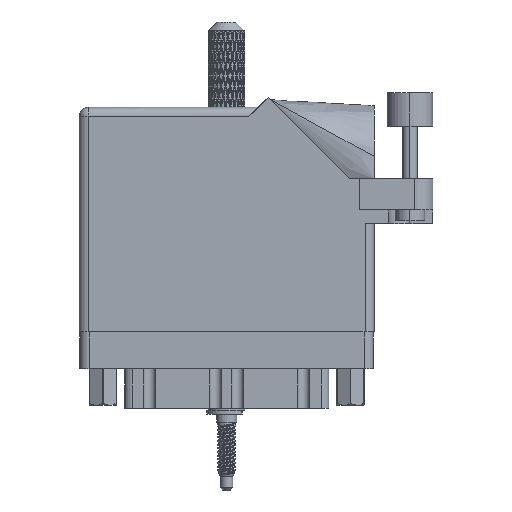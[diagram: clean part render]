
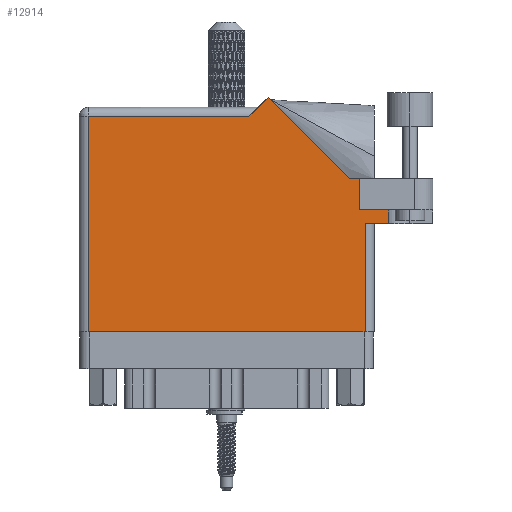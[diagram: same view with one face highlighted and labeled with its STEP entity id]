
A CAD part, front view. The second image highlights one B-rep face of the part: STEP entity #12914.
In plain terms, the highlighted face is planar.
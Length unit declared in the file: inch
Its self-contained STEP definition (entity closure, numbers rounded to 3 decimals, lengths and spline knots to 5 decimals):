
#301 = DIRECTION ( 'NONE',  ( 1., 0., 0. ) ) ;
#381 = ORIENTED_EDGE ( 'NONE', *, *, #11317, .T. ) ;
#4269 = CARTESIAN_POINT ( 'NONE',  ( 0., 1.53, 0. ) ) ;
#4334 = ORIENTED_EDGE ( 'NONE', *, *, #68360, .T. ) ;
#4575 = ORIENTED_EDGE ( 'NONE', *, *, #110889, .T. ) ;
#5026 = DIRECTION ( 'NONE',  ( 0., -1., 0. ) ) ;
#5050 = DIRECTION ( 'NONE',  ( 0., -1., 0. ) ) ;
#5153 = ORIENTED_EDGE ( 'NONE', *, *, #79553, .T. ) ;
#5802 = ORIENTED_EDGE ( 'NONE', *, *, #62195, .T. ) ;
#7744 = DIRECTION ( 'NONE',  ( -1., 0., 0. ) ) ;
#8622 = CARTESIAN_POINT ( 'NONE',  ( 0.062, 0., 0. ) ) ;
#9387 = DIRECTION ( 'NONE',  ( 0., 1., 0. ) ) ;
#10222 = ORIENTED_EDGE ( 'NONE', *, *, #43033, .F. ) ;
#10586 = DIRECTION ( 'NONE',  ( 0., 0., -1. ) ) ;
#11130 = CARTESIAN_POINT ( 'NONE',  ( 2.1115, 0.737, 0. ) ) ;
#11317 = EDGE_CURVE ( 'NONE', #102012, #17183, #24519, .T. ) ;
#11577 = VECTOR ( 'NONE', #9387, 39.37008 ) ;
#11699 = VERTEX_POINT ( 'NONE', #77248 ) ;
#12588 = DIRECTION ( 'NONE',  ( 0., 1., 0. ) ) ;
#12914 = ADVANCED_FACE ( 'NONE', ( #55962 ), #21453, .F. ) ;
#13253 = VECTOR ( 'NONE', #5026, 39.37008 ) ;
#14575 = VERTEX_POINT ( 'NONE', #109642 ) ;
#15927 = CARTESIAN_POINT ( 'NONE',  ( 0.062, 1.468, 0. ) ) ;
#17110 = VERTEX_POINT ( 'NONE', #109288 ) ;
#17183 = VERTEX_POINT ( 'NONE', #22547 ) ;
#17669 = ORIENTED_EDGE ( 'NONE', *, *, #80938, .T. ) ;
#18064 = LINE ( 'NONE', #88179, #62776 ) ;
#20840 = ORIENTED_EDGE ( 'NONE', *, *, #104533, .T. ) ;
#21453 = PLANE ( 'NONE',  #67649 ) ;
#22547 = CARTESIAN_POINT ( 'NONE',  ( 1.28771, 1.60071, 0. ) ) ;
#24519 = LINE ( 'NONE', #77959, #91090 ) ;
#24893 = VERTEX_POINT ( 'NONE', #15927 ) ;
#27526 = CARTESIAN_POINT ( 'NONE',  ( 1.91, 0.831, 0. ) ) ;
#28777 = CARTESIAN_POINT ( 'NONE',  ( 0., 1.468, 0. ) ) ;
#29037 = VECTOR ( 'NONE', #12588, 39.37008 ) ;
#30814 = VERTEX_POINT ( 'NONE', #96985 ) ;
#32569 = LINE ( 'NONE', #83734, #13253 ) ;
#33203 = VECTOR ( 'NONE', #73877, 39.37008 ) ;
#39583 = VERTEX_POINT ( 'NONE', #83125 ) ;
#40537 = ORIENTED_EDGE ( 'NONE', *, *, #44962, .F. ) ;
#41315 = CARTESIAN_POINT ( 'NONE',  ( 2.1115, 0.831, 0. ) ) ;
#43033 = EDGE_CURVE ( 'NONE', #39583, #92828, #108343, .T. ) ;
#44478 = EDGE_CURVE ( 'NONE', #17110, #24893, #51966, .T. ) ;
#44962 = EDGE_CURVE ( 'NONE', #92828, #45665, #57334, .T. ) ;
#45626 = DIRECTION ( 'NONE',  ( -1., 0., 0. ) ) ;
#45665 = VERTEX_POINT ( 'NONE', #11130 ) ;
#50397 = DIRECTION ( 'NONE',  ( -0.707, 0.707, 0. ) ) ;
#51966 = LINE ( 'NONE', #28777, #95375 ) ;
#52319 = ORIENTED_EDGE ( 'NONE', *, *, #104492, .T. ) ;
#52561 = LINE ( 'NONE', #78975, #82946 ) ;
#54319 = DIRECTION ( 'NONE',  ( 1., 0., 0. ) ) ;
#55962 = FACE_OUTER_BOUND ( 'NONE', #65599, .T. ) ;
#56877 = VECTOR ( 'NONE', #5050, 39.37008 ) ;
#56934 = DIRECTION ( 'NONE',  ( -1., 0., 0. ) ) ;
#57334 = LINE ( 'NONE', #83758, #56877 ) ;
#57964 = CARTESIAN_POINT ( 'NONE',  ( 1.948, 0.737, 0. ) ) ;
#61784 = LINE ( 'NONE', #105471, #105283 ) ;
#62195 = EDGE_CURVE ( 'NONE', #30814, #45665, #61784, .T. ) ;
#62776 = VECTOR ( 'NONE', #89857, 39.37008 ) ;
#64302 = VERTEX_POINT ( 'NONE', #8622 ) ;
#65599 = EDGE_LOOP ( 'NONE', ( #52319, #17669, #5802, #40537, #10222, #4575, #5153, #381, #20840, #87745, #4334 ) ) ;
#67649 = AXIS2_PLACEMENT_3D ( 'NONE', #4269, #10586, #45626 ) ;
#68360 = EDGE_CURVE ( 'NONE', #24893, #64302, #32569, .T. ) ;
#69312 = VECTOR ( 'NONE', #56934, 39.37008 ) ;
#72001 = CARTESIAN_POINT ( 'NONE',  ( 1.91, 0.831, 0. ) ) ;
#72516 = CARTESIAN_POINT ( 'NONE',  ( 2.41, 1.044, 0. ) ) ;
#73877 = DIRECTION ( 'NONE',  ( 1., 0., 0. ) ) ;
#77248 = CARTESIAN_POINT ( 'NONE',  ( 1.91, 1.044, 0. ) ) ;
#77959 = CARTESIAN_POINT ( 'NONE',  ( 1.84442, 1.044, 0. ) ) ;
#78336 = LINE ( 'NONE', #72001, #11577 ) ;
#78975 = CARTESIAN_POINT ( 'NONE',  ( 0., 0., 0. ) ) ;
#79553 = EDGE_CURVE ( 'NONE', #11699, #102012, #98907, .T. ) ;
#80938 = EDGE_CURVE ( 'NONE', #14575, #30814, #102175, .T. ) ;
#82946 = VECTOR ( 'NONE', #301, 39.37008 ) ;
#83125 = CARTESIAN_POINT ( 'NONE',  ( 1.91, 0.831, 0. ) ) ;
#83734 = CARTESIAN_POINT ( 'NONE',  ( 0.062, 0., 0. ) ) ;
#83758 = CARTESIAN_POINT ( 'NONE',  ( 2.1115, 1.16177, 0. ) ) ;
#87745 = ORIENTED_EDGE ( 'NONE', *, *, #44478, .T. ) ;
#88179 = CARTESIAN_POINT ( 'NONE',  ( 1.217, 1.53, 0. ) ) ;
#89857 = DIRECTION ( 'NONE',  ( -0.707, -0.707, 0. ) ) ;
#91090 = VECTOR ( 'NONE', #50397, 39.37008 ) ;
#92828 = VERTEX_POINT ( 'NONE', #41315 ) ;
#95375 = VECTOR ( 'NONE', #7744, 39.37008 ) ;
#96985 = CARTESIAN_POINT ( 'NONE',  ( 1.948, 0.737, 0. ) ) ;
#97348 = CARTESIAN_POINT ( 'NONE',  ( 1.84442, 1.044, 0. ) ) ;
#98907 = LINE ( 'NONE', #72516, #69312 ) ;
#102012 = VERTEX_POINT ( 'NONE', #97348 ) ;
#102175 = LINE ( 'NONE', #57964, #29037 ) ;
#104492 = EDGE_CURVE ( 'NONE', #64302, #14575, #52561, .T. ) ;
#104533 = EDGE_CURVE ( 'NONE', #17183, #17110, #18064, .T. ) ;
#105283 = VECTOR ( 'NONE', #54319, 39.37008 ) ;
#105471 = CARTESIAN_POINT ( 'NONE',  ( 2.01, 0.737, 0. ) ) ;
#108343 = LINE ( 'NONE', #27526, #33203 ) ;
#109288 = CARTESIAN_POINT ( 'NONE',  ( 1.155, 1.468, 0. ) ) ;
#109642 = CARTESIAN_POINT ( 'NONE',  ( 1.948, 0., 0. ) ) ;
#110889 = EDGE_CURVE ( 'NONE', #39583, #11699, #78336, .T. ) ;
